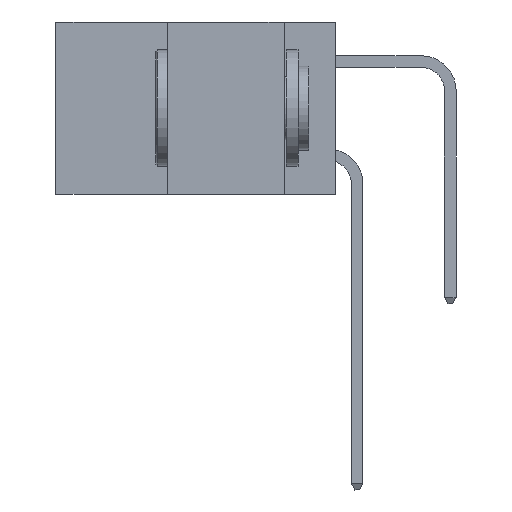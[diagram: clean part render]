
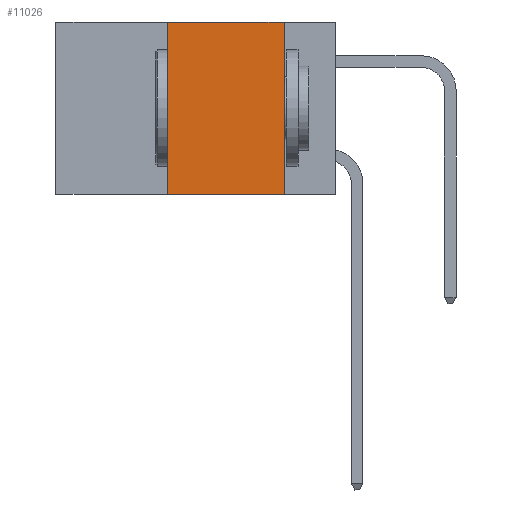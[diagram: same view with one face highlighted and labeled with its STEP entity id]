
A CAD part, left-side view. The second image highlights one B-rep face of the part: STEP entity #11026.
In plain terms, the highlighted planar face has unit normal (-1, 0, 0).
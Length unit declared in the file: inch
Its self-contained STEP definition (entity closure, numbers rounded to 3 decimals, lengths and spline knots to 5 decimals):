
#711 = VERTEX_POINT ( 'NONE', #2472 ) ;
#1165 = LINE ( 'NONE', #3055, #4217 ) ;
#1447 = VERTEX_POINT ( 'NONE', #3988 ) ;
#1583 = VERTEX_POINT ( 'NONE', #6966 ) ;
#1964 = DIRECTION ( 'NONE',  ( 0., 0., -1. ) ) ;
#2472 = CARTESIAN_POINT ( 'NONE',  ( 0., 0.36, -0.37 ) ) ;
#2481 = EDGE_CURVE ( 'NONE', #1583, #1447, #1165, .T. ) ;
#2565 = CARTESIAN_POINT ( 'NONE',  ( 0., 0.11, -0.37 ) ) ;
#2884 = CARTESIAN_POINT ( 'NONE',  ( 0., 0.11, 0. ) ) ;
#3055 = CARTESIAN_POINT ( 'NONE',  ( 0., 0.6, 0. ) ) ;
#3087 = VECTOR ( 'NONE', #1964, 39.37008 ) ;
#3633 = EDGE_CURVE ( 'NONE', #711, #1583, #7406, .T. ) ;
#3673 = DIRECTION ( 'NONE',  ( 0., 0., -1. ) ) ;
#3988 = CARTESIAN_POINT ( 'NONE',  ( 0., 0.11, 0. ) ) ;
#4182 = CARTESIAN_POINT ( 'NONE',  ( 0., 0.6, -0.37 ) ) ;
#4217 = VECTOR ( 'NONE', #9749, 39.37008 ) ;
#5273 = ORIENTED_EDGE ( 'NONE', *, *, #3633, .F. ) ;
#5561 = CARTESIAN_POINT ( 'NONE',  ( 0., 0.6, 0. ) ) ;
#5988 = DIRECTION ( 'NONE',  ( 0., 0., 1. ) ) ;
#6646 = PLANE ( 'NONE',  #8508 ) ;
#6966 = CARTESIAN_POINT ( 'NONE',  ( 0., 0.36, 0. ) ) ;
#7171 = FACE_OUTER_BOUND ( 'NONE', #8424, .T. ) ;
#7406 = LINE ( 'NONE', #9952, #11549 ) ;
#7919 = ORIENTED_EDGE ( 'NONE', *, *, #2481, .F. ) ;
#8424 = EDGE_LOOP ( 'NONE', ( #8819, #7919, #5273, #11434 ) ) ;
#8508 = AXIS2_PLACEMENT_3D ( 'NONE', #5561, #12505, #3673 ) ;
#8594 = LINE ( 'NONE', #2884, #3087 ) ;
#8819 = ORIENTED_EDGE ( 'NONE', *, *, #8896, .F. ) ;
#8896 = EDGE_CURVE ( 'NONE', #1447, #9083, #8594, .T. ) ;
#9083 = VERTEX_POINT ( 'NONE', #2565 ) ;
#9193 = LINE ( 'NONE', #4182, #11327 ) ;
#9749 = DIRECTION ( 'NONE',  ( 0., -1., 0. ) ) ;
#9952 = CARTESIAN_POINT ( 'NONE',  ( 0., 0.36, 0. ) ) ;
#10077 = EDGE_CURVE ( 'NONE', #711, #9083, #9193, .T. ) ;
#11026 = ADVANCED_FACE ( 'NONE', ( #7171 ), #6646, .F. ) ;
#11327 = VECTOR ( 'NONE', #12007, 39.37008 ) ;
#11434 = ORIENTED_EDGE ( 'NONE', *, *, #10077, .T. ) ;
#11549 = VECTOR ( 'NONE', #5988, 39.37008 ) ;
#12007 = DIRECTION ( 'NONE',  ( 0., -1., 0. ) ) ;
#12505 = DIRECTION ( 'NONE',  ( 1., 0., 0. ) ) ;
